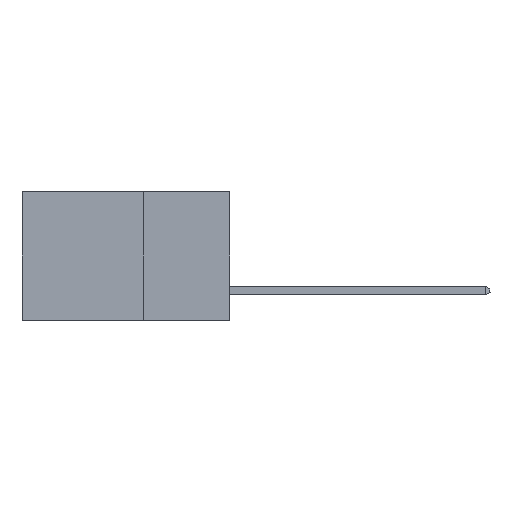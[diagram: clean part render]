
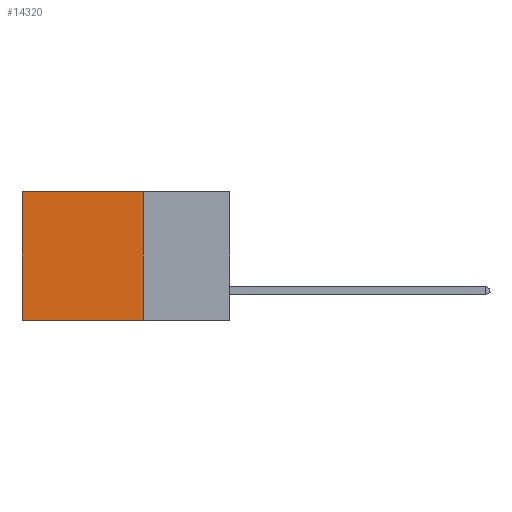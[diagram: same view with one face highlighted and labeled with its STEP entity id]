
A CAD part, left-side view. The second image highlights one B-rep face of the part: STEP entity #14320.
In plain terms, the highlighted planar face has unit normal (-1, 0, 0).
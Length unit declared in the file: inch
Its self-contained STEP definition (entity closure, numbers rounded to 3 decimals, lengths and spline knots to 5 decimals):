
#214 = EDGE_CURVE ( 'NONE', #308, #13914, #11697, .T. ) ;
#308 = VERTEX_POINT ( 'NONE', #1361 ) ;
#422 = EDGE_CURVE ( 'NONE', #308, #3867, #3512, .T. ) ;
#1361 = CARTESIAN_POINT ( 'NONE',  ( 0.298, 0.25, 0. ) ) ;
#1493 = VECTOR ( 'NONE', #10908, 39.37008 ) ;
#1517 = VECTOR ( 'NONE', #3810, 39.37008 ) ;
#1650 = EDGE_LOOP ( 'NONE', ( #14764, #3302, #15366, #12205 ) ) ;
#1723 = DIRECTION ( 'NONE',  ( 0., 1., 0. ) ) ;
#2333 = DIRECTION ( 'NONE',  ( 0., 1., 0. ) ) ;
#3302 = ORIENTED_EDGE ( 'NONE', *, *, #8880, .F. ) ;
#3311 = PLANE ( 'NONE',  #7756 ) ;
#3512 = LINE ( 'NONE', #6249, #1517 ) ;
#3810 = DIRECTION ( 'NONE',  ( 0., 0., -1. ) ) ;
#3867 = VERTEX_POINT ( 'NONE', #13522 ) ;
#4627 = DIRECTION ( 'NONE',  ( 1., 0., 0. ) ) ;
#4699 = CARTESIAN_POINT ( 'NONE',  ( 0.298, 0.25, 0. ) ) ;
#4949 = VECTOR ( 'NONE', #2333, 39.37008 ) ;
#6249 = CARTESIAN_POINT ( 'NONE',  ( 0.298, 0.25, 0. ) ) ;
#6273 = VERTEX_POINT ( 'NONE', #16509 ) ;
#6874 = CARTESIAN_POINT ( 'NONE',  ( 0.298, 0.6, 0. ) ) ;
#7756 = AXIS2_PLACEMENT_3D ( 'NONE', #14692, #4627, #14812 ) ;
#7972 = CARTESIAN_POINT ( 'NONE',  ( 0.298, 0.25, -0.37 ) ) ;
#8880 = EDGE_CURVE ( 'NONE', #3867, #6273, #16103, .T. ) ;
#9337 = VECTOR ( 'NONE', #1723, 39.37008 ) ;
#10908 = DIRECTION ( 'NONE',  ( 0., 0., -1. ) ) ;
#11697 = LINE ( 'NONE', #4699, #4949 ) ;
#12205 = ORIENTED_EDGE ( 'NONE', *, *, #214, .T. ) ;
#12452 = FACE_OUTER_BOUND ( 'NONE', #1650, .T. ) ;
#13522 = CARTESIAN_POINT ( 'NONE',  ( 0.298, 0.25, -0.37 ) ) ;
#13662 = CARTESIAN_POINT ( 'NONE',  ( 0.298, 0.6, 0. ) ) ;
#13914 = VERTEX_POINT ( 'NONE', #13662 ) ;
#14175 = EDGE_CURVE ( 'NONE', #13914, #6273, #15029, .T. ) ;
#14320 = ADVANCED_FACE ( 'NONE', ( #12452 ), #3311, .F. ) ;
#14692 = CARTESIAN_POINT ( 'NONE',  ( 0.298, 0.25, 0. ) ) ;
#14764 = ORIENTED_EDGE ( 'NONE', *, *, #14175, .T. ) ;
#14812 = DIRECTION ( 'NONE',  ( 0., 0., -1. ) ) ;
#15029 = LINE ( 'NONE', #6874, #1493 ) ;
#15366 = ORIENTED_EDGE ( 'NONE', *, *, #422, .F. ) ;
#16103 = LINE ( 'NONE', #7972, #9337 ) ;
#16509 = CARTESIAN_POINT ( 'NONE',  ( 0.298, 0.6, -0.37 ) ) ;
